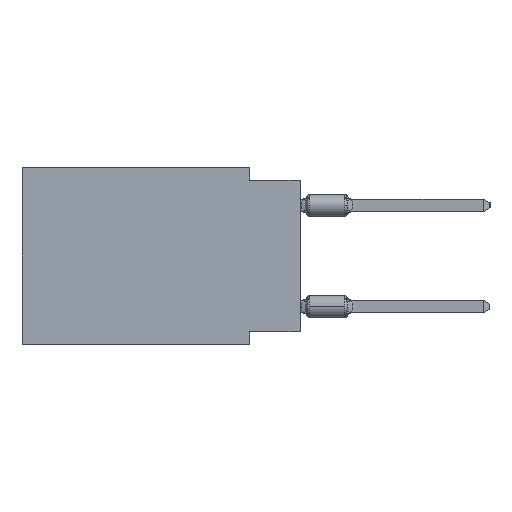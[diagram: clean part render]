
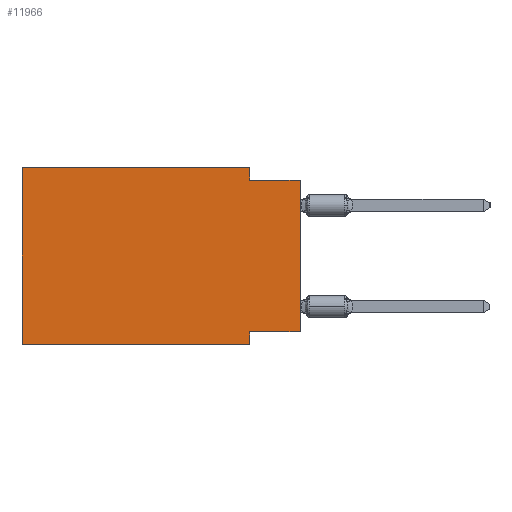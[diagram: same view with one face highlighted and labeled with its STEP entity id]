
A CAD part, left-side view. The second image highlights one B-rep face of the part: STEP entity #11966.
In plain terms, the highlighted planar face has unit normal (-1, 0, 0).
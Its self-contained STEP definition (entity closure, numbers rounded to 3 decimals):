
#807 = VERTEX_POINT ( 'NONE', #36088 ) ;
#1166 = VECTOR ( 'NONE', #23954, 1000. ) ;
#2671 = CARTESIAN_POINT ( 'NONE',  ( 0., 0., -8.255 ) ) ;
#2683 = CARTESIAN_POINT ( 'NONE',  ( 0., 13.97, 0. ) ) ;
#2972 = CARTESIAN_POINT ( 'NONE',  ( 0., 2.54, -8.255 ) ) ;
#3858 = CARTESIAN_POINT ( 'NONE',  ( 0., 13.97, 0. ) ) ;
#5211 = DIRECTION ( 'NONE',  ( 0., -1., 0. ) ) ;
#5426 = ORIENTED_EDGE ( 'NONE', *, *, #15394, .F. ) ;
#7533 = CARTESIAN_POINT ( 'NONE',  ( 0., 2.54, 0. ) ) ;
#7919 = LINE ( 'NONE', #7533, #29965 ) ;
#8167 = EDGE_CURVE ( 'NONE', #17058, #807, #33042, .T. ) ;
#8285 = ORIENTED_EDGE ( 'NONE', *, *, #19323, .F. ) ;
#8386 = DIRECTION ( 'NONE',  ( 0., 0., -1. ) ) ;
#8517 = EDGE_LOOP ( 'NONE', ( #12073, #9069, #34013, #5426, #20939, #30171, #26798, #8285 ) ) ;
#9069 = ORIENTED_EDGE ( 'NONE', *, *, #12147, .F. ) ;
#9164 = DIRECTION ( 'NONE',  ( 0., -1., 0. ) ) ;
#9223 = VECTOR ( 'NONE', #28863, 1000. ) ;
#9573 = LINE ( 'NONE', #33147, #33159 ) ;
#10433 = DIRECTION ( 'NONE',  ( 0., 0., -1. ) ) ;
#11108 = FACE_OUTER_BOUND ( 'NONE', #8517, .T. ) ;
#11729 = VECTOR ( 'NONE', #20870, 1000. ) ;
#11966 = ADVANCED_FACE ( 'NONE', ( #11108 ), #34679, .F. ) ;
#12073 = ORIENTED_EDGE ( 'NONE', *, *, #20933, .T. ) ;
#12147 = EDGE_CURVE ( 'NONE', #19539, #17170, #15530, .T. ) ;
#13054 = CARTESIAN_POINT ( 'NONE',  ( 0., 2.54, -8.89 ) ) ;
#13280 = VECTOR ( 'NONE', #5211, 1000. ) ;
#13443 = CARTESIAN_POINT ( 'NONE',  ( 0., 0., 0. ) ) ;
#14003 = CARTESIAN_POINT ( 'NONE',  ( 0., 13.97, 0. ) ) ;
#15394 = EDGE_CURVE ( 'NONE', #807, #29158, #20291, .T. ) ;
#15530 = LINE ( 'NONE', #24418, #37256 ) ;
#15763 = LINE ( 'NONE', #13443, #1166 ) ;
#17058 = VERTEX_POINT ( 'NONE', #31716 ) ;
#17170 = VERTEX_POINT ( 'NONE', #26492 ) ;
#17847 = CARTESIAN_POINT ( 'NONE',  ( 0., 2.54, -0.635 ) ) ;
#18506 = CARTESIAN_POINT ( 'NONE',  ( 0., 2.54, -8.89 ) ) ;
#19323 = EDGE_CURVE ( 'NONE', #28474, #31841, #9573, .T. ) ;
#19539 = VERTEX_POINT ( 'NONE', #17847 ) ;
#20291 = LINE ( 'NONE', #2683, #13280 ) ;
#20410 = CARTESIAN_POINT ( 'NONE',  ( 0., 2.54, 0. ) ) ;
#20870 = DIRECTION ( 'NONE',  ( 0., 0., 1. ) ) ;
#20933 = EDGE_CURVE ( 'NONE', #28474, #17170, #15763, .T. ) ;
#20939 = ORIENTED_EDGE ( 'NONE', *, *, #8167, .F. ) ;
#21479 = EDGE_CURVE ( 'NONE', #17058, #34643, #30809, .T. ) ;
#23954 = DIRECTION ( 'NONE',  ( 0., 0., 1. ) ) ;
#24418 = CARTESIAN_POINT ( 'NONE',  ( 0., 0., -0.635 ) ) ;
#26138 = AXIS2_PLACEMENT_3D ( 'NONE', #14003, #31974, #8386 ) ;
#26492 = CARTESIAN_POINT ( 'NONE',  ( 0., 0., -0.635 ) ) ;
#26798 = ORIENTED_EDGE ( 'NONE', *, *, #28763, .F. ) ;
#27792 = DIRECTION ( 'NONE',  ( 0., 0., -1. ) ) ;
#28302 = CARTESIAN_POINT ( 'NONE',  ( 0., 13.97, -8.89 ) ) ;
#28474 = VERTEX_POINT ( 'NONE', #2671 ) ;
#28763 = EDGE_CURVE ( 'NONE', #31841, #34643, #30491, .T. ) ;
#28863 = DIRECTION ( 'NONE',  ( 0., -1., 0. ) ) ;
#29158 = VERTEX_POINT ( 'NONE', #20410 ) ;
#29574 = VECTOR ( 'NONE', #27792, 1000. ) ;
#29965 = VECTOR ( 'NONE', #10433, 1000. ) ;
#30171 = ORIENTED_EDGE ( 'NONE', *, *, #21479, .T. ) ;
#30491 = LINE ( 'NONE', #18506, #29574 ) ;
#30809 = LINE ( 'NONE', #28302, #9223 ) ;
#31716 = CARTESIAN_POINT ( 'NONE',  ( 0., 13.97, -8.89 ) ) ;
#31841 = VERTEX_POINT ( 'NONE', #2972 ) ;
#31974 = DIRECTION ( 'NONE',  ( 1., 0., 0. ) ) ;
#33042 = LINE ( 'NONE', #3858, #11729 ) ;
#33147 = CARTESIAN_POINT ( 'NONE',  ( 0., 0., -8.255 ) ) ;
#33159 = VECTOR ( 'NONE', #37180, 1000. ) ;
#34013 = ORIENTED_EDGE ( 'NONE', *, *, #37463, .F. ) ;
#34643 = VERTEX_POINT ( 'NONE', #13054 ) ;
#34679 = PLANE ( 'NONE',  #26138 ) ;
#36088 = CARTESIAN_POINT ( 'NONE',  ( 0., 13.97, 0. ) ) ;
#37180 = DIRECTION ( 'NONE',  ( 0., 1., 0. ) ) ;
#37256 = VECTOR ( 'NONE', #9164, 1000. ) ;
#37463 = EDGE_CURVE ( 'NONE', #29158, #19539, #7919, .T. ) ;
